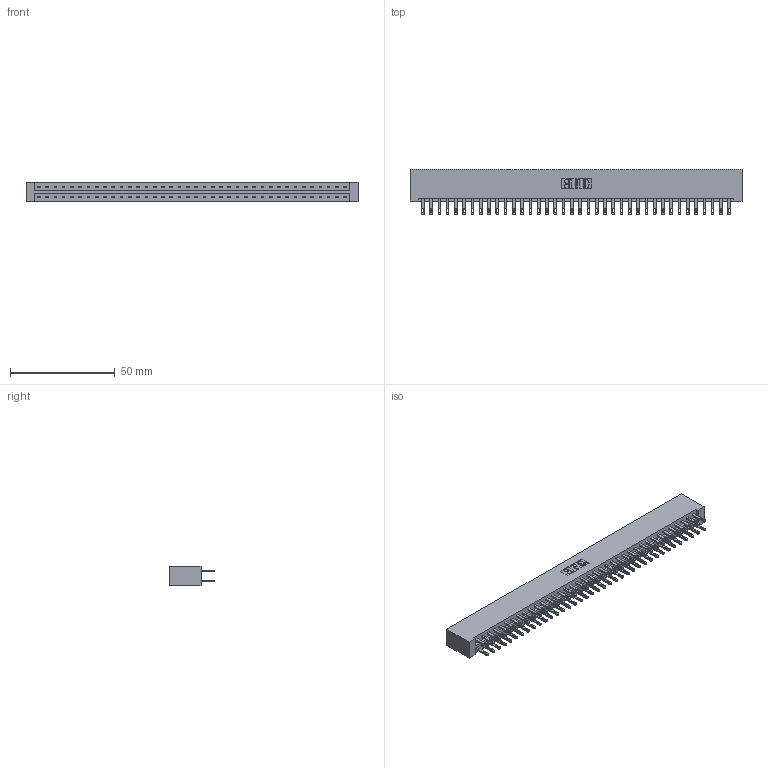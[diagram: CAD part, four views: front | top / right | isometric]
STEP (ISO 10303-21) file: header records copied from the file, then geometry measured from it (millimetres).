
FILE_DESCRIPTION (( 'STEP AP203' ), '1' );
FILE_NAME ('833-076-500-201.STEP', '2020-06-05T17:40:43', ( '' ), ( '' ), 'SwSTEP 2.0', 'SolidWorks 2020', '' );
FILE_SCHEMA (( 'CONFIG_CONTROL_DESIGN' ));
Length unit declared in the file: inch
Products named in the file (3): 833 Part_Lugless; 345-292-001_345-293-100; 833-076-500-201
Assembly tree (77 placements, depth 2):
  833-076-500-201
    833 Part_Lugless
    345-292-001_345-293-100  x76
Bounding box: 158.83 x 21.85 x 9.4 mm (x, y, z)
Volume: 17042.3 mm3; surface area: 20966 mm2
Topology: 77 solids, 77 shells, 3754 faces, 11459 edges, 7638 vertices
Faces by surface type: plane 2346, cylinder 1408
Entity records: 24617 total; most frequent: CARTESIAN_POINT 4082, ORIENTED_EDGE 4018, DIRECTION 3489, EDGE_CURVE 2009, LINE 1885, VECTOR 1885, VERTEX_POINT 1338, AXIS2_PLACEMENT_3D 802
